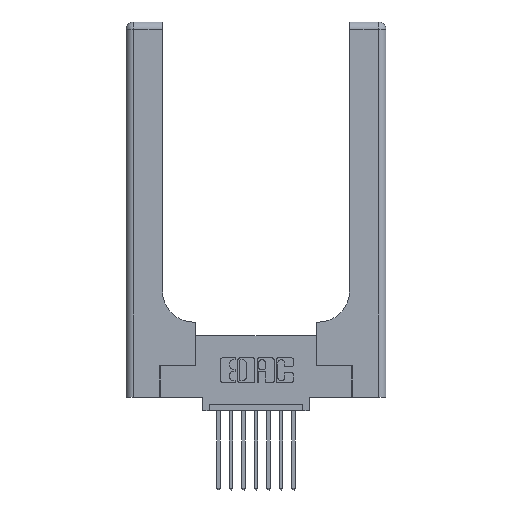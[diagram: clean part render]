
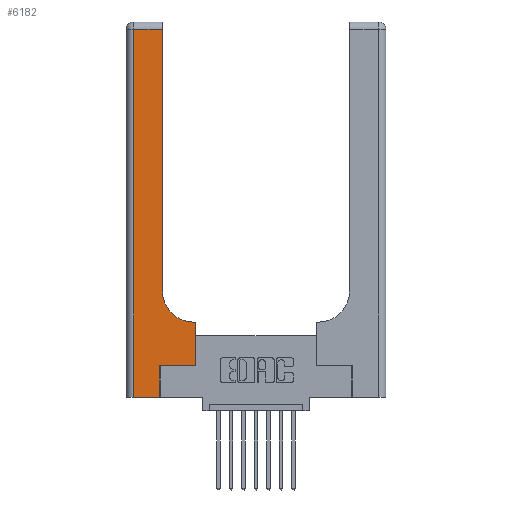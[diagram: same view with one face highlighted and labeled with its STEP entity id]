
A CAD part, top view. The second image highlights one B-rep face of the part: STEP entity #6182.
In plain terms, the highlighted planar face has unit normal (0, 0, 1).
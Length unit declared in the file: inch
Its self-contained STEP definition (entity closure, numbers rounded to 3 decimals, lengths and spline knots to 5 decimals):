
#82 = VERTEX_POINT ( 'NONE', #9532 ) ;
#189 = CARTESIAN_POINT ( 'NONE',  ( 0.5415, 0.6, 0.37 ) ) ;
#710 = EDGE_CURVE ( 'NONE', #2187, #7565, #9478, .T. ) ;
#972 = ORIENTED_EDGE ( 'NONE', *, *, #7516, .T. ) ;
#976 = DIRECTION ( 'NONE',  ( 0., 1., 0. ) ) ;
#1292 = ORIENTED_EDGE ( 'NONE', *, *, #5676, .T. ) ;
#1322 = CARTESIAN_POINT ( 'NONE',  ( 0.06, 0., 0.37 ) ) ;
#1331 = EDGE_CURVE ( 'NONE', #13945, #82, #8799, .T. ) ;
#1385 = VERTEX_POINT ( 'NONE', #2667 ) ;
#1516 = EDGE_CURVE ( 'NONE', #7565, #13945, #8408, .T. ) ;
#1640 = DIRECTION ( 'NONE',  ( 0., 1., 0. ) ) ;
#1714 = EDGE_CURVE ( 'NONE', #4748, #2187, #5623, .T. ) ;
#2187 = VERTEX_POINT ( 'NONE', #1322 ) ;
#2435 = ORIENTED_EDGE ( 'NONE', *, *, #1714, .T. ) ;
#2463 = DIRECTION ( 'NONE',  ( 1., 0., 0. ) ) ;
#2667 = CARTESIAN_POINT ( 'NONE',  ( 0.5585, 0.6, 0.37 ) ) ;
#4006 = EDGE_LOOP ( 'NONE', ( #972, #1292, #2435, #14583, #8878, #4137, #7627, #13988, #8382 ) ) ;
#4137 = ORIENTED_EDGE ( 'NONE', *, *, #1331, .T. ) ;
#4140 = VECTOR ( 'NONE', #9982, 39.37008 ) ;
#4485 = AXIS2_PLACEMENT_3D ( 'NONE', #15077, #11641, #7982 ) ;
#4710 = CARTESIAN_POINT ( 'NONE',  ( 0.269, 0.25, 0.37 ) ) ;
#4748 = VERTEX_POINT ( 'NONE', #10104 ) ;
#4800 = DIRECTION ( 'NONE',  ( -1., 0., 0. ) ) ;
#5449 = VECTOR ( 'NONE', #976, 39.37008 ) ;
#5604 = LINE ( 'NONE', #11193, #4140 ) ;
#5623 = LINE ( 'NONE', #9204, #9881 ) ;
#5667 = FACE_OUTER_BOUND ( 'NONE', #4006, .T. ) ;
#5676 = EDGE_CURVE ( 'NONE', #13080, #4748, #11838, .T. ) ;
#5799 = CARTESIAN_POINT ( 'NONE',  ( 0.269, 0., 0.37 ) ) ;
#6182 = ADVANCED_FACE ( 'NONE', ( #5667 ), #6596, .F. ) ;
#6231 = VERTEX_POINT ( 'NONE', #189 ) ;
#6596 = PLANE ( 'NONE',  #14388 ) ;
#6702 = VECTOR ( 'NONE', #8110, 39.37008 ) ;
#6824 = CIRCLE ( 'NONE', #4485, 0.25 ) ;
#7125 = CARTESIAN_POINT ( 'NONE',  ( 0., 0., 0.37 ) ) ;
#7516 = EDGE_CURVE ( 'NONE', #14954, #13080, #12335, .T. ) ;
#7565 = VERTEX_POINT ( 'NONE', #10049 ) ;
#7627 = ORIENTED_EDGE ( 'NONE', *, *, #9540, .T. ) ;
#7830 = EDGE_CURVE ( 'NONE', #6231, #14954, #6824, .T. ) ;
#7982 = DIRECTION ( 'NONE',  ( 1., 0., 0. ) ) ;
#8110 = DIRECTION ( 'NONE',  ( 1., 0., 0. ) ) ;
#8247 = VECTOR ( 'NONE', #1640, 39.37008 ) ;
#8382 = ORIENTED_EDGE ( 'NONE', *, *, #7830, .T. ) ;
#8408 = LINE ( 'NONE', #5799, #5449 ) ;
#8519 = CARTESIAN_POINT ( 'NONE',  ( 0., 2.94, 0.37 ) ) ;
#8675 = VECTOR ( 'NONE', #8682, 39.37008 ) ;
#8682 = DIRECTION ( 'NONE',  ( -1., 0., 0. ) ) ;
#8799 = LINE ( 'NONE', #4710, #13446 ) ;
#8878 = ORIENTED_EDGE ( 'NONE', *, *, #1516, .T. ) ;
#9204 = CARTESIAN_POINT ( 'NONE',  ( 0.06, 3., 0.37 ) ) ;
#9478 = LINE ( 'NONE', #7125, #6702 ) ;
#9532 = CARTESIAN_POINT ( 'NONE',  ( 0.5585, 0.25, 0.37 ) ) ;
#9540 = EDGE_CURVE ( 'NONE', #82, #1385, #11228, .T. ) ;
#9592 = DIRECTION ( 'NONE',  ( 0., 0., -1. ) ) ;
#9881 = VECTOR ( 'NONE', #12777, 39.37008 ) ;
#9982 = DIRECTION ( 'NONE',  ( -1., 0., 0. ) ) ;
#10049 = CARTESIAN_POINT ( 'NONE',  ( 0.269, 0., 0.37 ) ) ;
#10104 = CARTESIAN_POINT ( 'NONE',  ( 0.06, 2.94, 0.37 ) ) ;
#10125 = CARTESIAN_POINT ( 'NONE',  ( 0., 3., 0.37 ) ) ;
#10295 = VECTOR ( 'NONE', #10988, 39.37008 ) ;
#10988 = DIRECTION ( 'NONE',  ( 0., 1., 0. ) ) ;
#11193 = CARTESIAN_POINT ( 'NONE',  ( 0.2915, 0.6, 0.37 ) ) ;
#11228 = LINE ( 'NONE', #13488, #10295 ) ;
#11641 = DIRECTION ( 'NONE',  ( 0., 0., -1. ) ) ;
#11838 = LINE ( 'NONE', #8519, #8675 ) ;
#11865 = EDGE_CURVE ( 'NONE', #1385, #6231, #5604, .T. ) ;
#12010 = CARTESIAN_POINT ( 'NONE',  ( 0.2915, 0.85, 0.37 ) ) ;
#12300 = CARTESIAN_POINT ( 'NONE',  ( 0.2915, 3., 0.37 ) ) ;
#12335 = LINE ( 'NONE', #12300, #8247 ) ;
#12777 = DIRECTION ( 'NONE',  ( 0., -1., 0. ) ) ;
#13080 = VERTEX_POINT ( 'NONE', #14868 ) ;
#13200 = CARTESIAN_POINT ( 'NONE',  ( 0.269, 0.25, 0.37 ) ) ;
#13446 = VECTOR ( 'NONE', #2463, 39.37008 ) ;
#13488 = CARTESIAN_POINT ( 'NONE',  ( 0.5585, 0.25, 0.37 ) ) ;
#13945 = VERTEX_POINT ( 'NONE', #13200 ) ;
#13988 = ORIENTED_EDGE ( 'NONE', *, *, #11865, .T. ) ;
#14388 = AXIS2_PLACEMENT_3D ( 'NONE', #10125, #9592, #4800 ) ;
#14583 = ORIENTED_EDGE ( 'NONE', *, *, #710, .T. ) ;
#14868 = CARTESIAN_POINT ( 'NONE',  ( 0.2915, 2.94, 0.37 ) ) ;
#14954 = VERTEX_POINT ( 'NONE', #12010 ) ;
#15077 = CARTESIAN_POINT ( 'NONE',  ( 0.5415, 0.85, 0.37 ) ) ;
